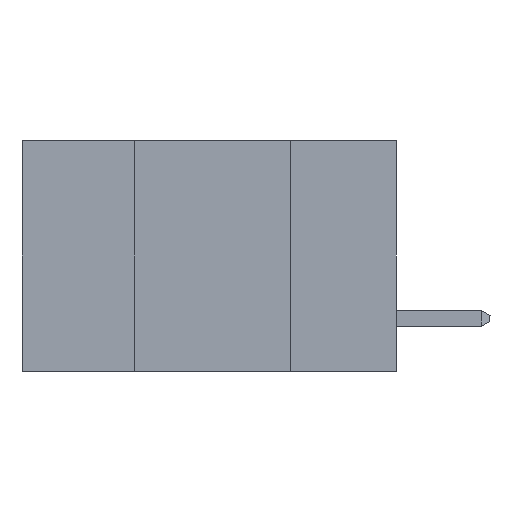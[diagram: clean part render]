
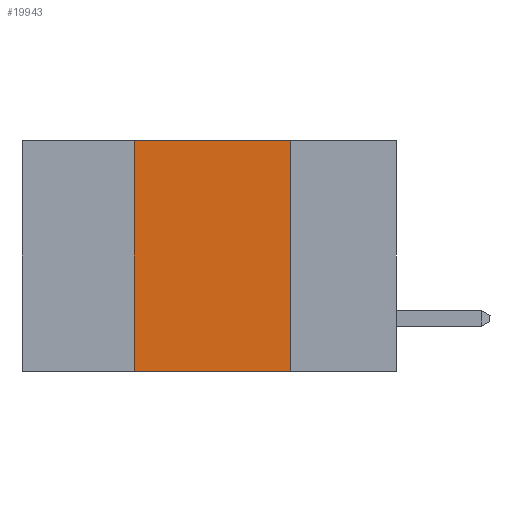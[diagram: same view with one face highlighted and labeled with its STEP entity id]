
A CAD part, left-side view. The second image highlights one B-rep face of the part: STEP entity #19943.
In plain terms, the highlighted planar face has unit normal (-1, 0, 0).
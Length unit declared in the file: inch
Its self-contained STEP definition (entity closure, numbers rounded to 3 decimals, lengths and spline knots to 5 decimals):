
#1165 = FACE_OUTER_BOUND ( 'NONE', #16967, .T. ) ;
#1585 = CARTESIAN_POINT ( 'NONE',  ( 0., 0.6, 0. ) ) ;
#2344 = ORIENTED_EDGE ( 'NONE', *, *, #16373, .F. ) ;
#2696 = VERTEX_POINT ( 'NONE', #3945 ) ;
#2947 = PLANE ( 'NONE',  #20336 ) ;
#3707 = CARTESIAN_POINT ( 'NONE',  ( 0., 0.6, -0.37 ) ) ;
#3945 = CARTESIAN_POINT ( 'NONE',  ( 0., 0.42, 0. ) ) ;
#4124 = CARTESIAN_POINT ( 'NONE',  ( 0., 0.42, -0.37 ) ) ;
#4888 = DIRECTION ( 'NONE',  ( 0., -1., 0. ) ) ;
#5330 = ORIENTED_EDGE ( 'NONE', *, *, #14361, .F. ) ;
#5566 = ORIENTED_EDGE ( 'NONE', *, *, #15009, .T. ) ;
#5900 = LINE ( 'NONE', #12547, #6245 ) ;
#5980 = DIRECTION ( 'NONE',  ( 1., 0., 0. ) ) ;
#6245 = VECTOR ( 'NONE', #18885, 39.37008 ) ;
#7428 = DIRECTION ( 'NONE',  ( 0., -1., 0. ) ) ;
#8004 = ORIENTED_EDGE ( 'NONE', *, *, #9258, .F. ) ;
#8059 = VECTOR ( 'NONE', #16818, 39.37008 ) ;
#8603 = VERTEX_POINT ( 'NONE', #17278 ) ;
#8825 = VECTOR ( 'NONE', #4888, 39.37008 ) ;
#9258 = EDGE_CURVE ( 'NONE', #11901, #2696, #11810, .T. ) ;
#10808 = CARTESIAN_POINT ( 'NONE',  ( 0., 0.42, -0.37 ) ) ;
#11810 = LINE ( 'NONE', #4124, #8059 ) ;
#11901 = VERTEX_POINT ( 'NONE', #10808 ) ;
#12547 = CARTESIAN_POINT ( 'NONE',  ( 0., 0.17, -0.37 ) ) ;
#13879 = DIRECTION ( 'NONE',  ( 0., 0., -1. ) ) ;
#14361 = EDGE_CURVE ( 'NONE', #2696, #8603, #17575, .T. ) ;
#15009 = EDGE_CURVE ( 'NONE', #11901, #15674, #16103, .T. ) ;
#15674 = VERTEX_POINT ( 'NONE', #20216 ) ;
#15860 = VECTOR ( 'NONE', #7428, 39.37008 ) ;
#16103 = LINE ( 'NONE', #3707, #8825 ) ;
#16373 = EDGE_CURVE ( 'NONE', #8603, #15674, #5900, .T. ) ;
#16818 = DIRECTION ( 'NONE',  ( 0., 0., 1. ) ) ;
#16967 = EDGE_LOOP ( 'NONE', ( #2344, #5330, #8004, #5566 ) ) ;
#17278 = CARTESIAN_POINT ( 'NONE',  ( 0., 0.17, 0. ) ) ;
#17575 = LINE ( 'NONE', #18945, #15860 ) ;
#18885 = DIRECTION ( 'NONE',  ( 0., 0., -1. ) ) ;
#18945 = CARTESIAN_POINT ( 'NONE',  ( 0., 0.6, 0. ) ) ;
#19943 = ADVANCED_FACE ( 'NONE', ( #1165 ), #2947, .F. ) ;
#20216 = CARTESIAN_POINT ( 'NONE',  ( 0., 0.17, -0.37 ) ) ;
#20336 = AXIS2_PLACEMENT_3D ( 'NONE', #1585, #5980, #13879 ) ;
